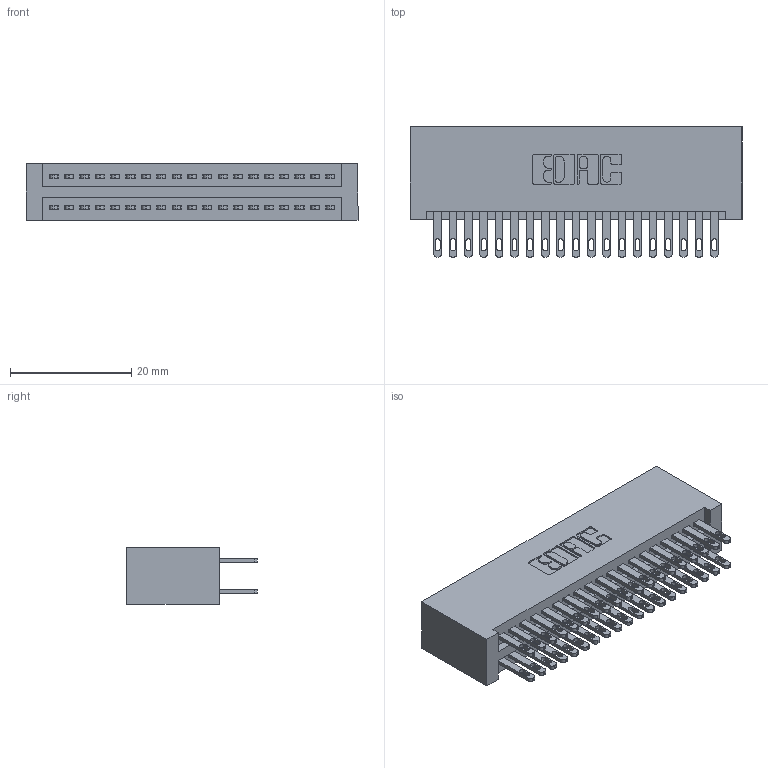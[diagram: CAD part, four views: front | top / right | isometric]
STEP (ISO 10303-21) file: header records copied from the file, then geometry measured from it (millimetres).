
FILE_DESCRIPTION (( 'STEP AP203' ), '1' );
FILE_NAME ('345-038-500-201.STEP', '2018-08-30T04:31:04', ( '' ), ( '' ), 'SwSTEP 2.0', 'SolidWorks 2016', '' );
FILE_SCHEMA (( 'CONFIG_CONTROL_DESIGN' ));
Length unit declared in the file: inch
Products named in the file (3): 345 Part_No Mounting Lugs; 345-292-001_345-293-100; 345-038-500-201
Assembly tree (39 placements, depth 2):
  345-038-500-201
    345 Part_No Mounting Lugs
    345-292-001_345-293-100  x38
Bounding box: 54.86 x 21.51 x 9.4 mm (x, y, z)
Volume: 5848.1 mm3; surface area: 8889.8 mm2
Topology: 39 solids, 39 shells, 1866 faces, 5675 edges, 3782 vertices
Faces by surface type: plane 1102, cylinder 764
Entity records: 17657 total; most frequent: CARTESIAN_POINT 2980, ORIENTED_EDGE 2914, DIRECTION 2653, EDGE_CURVE 1457, VECTOR 1253, LINE 1253, VERTEX_POINT 970, AXIS2_PLACEMENT_3D 700
